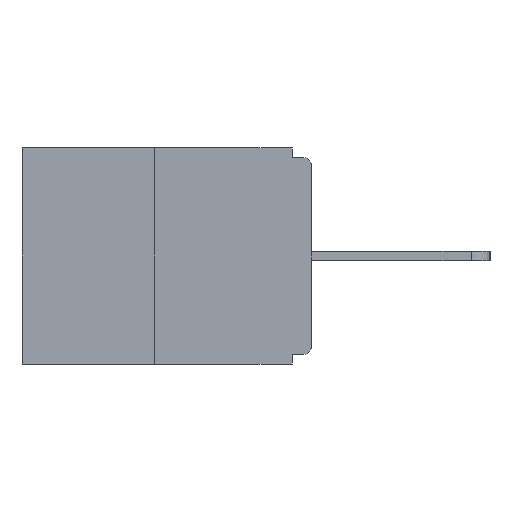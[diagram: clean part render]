
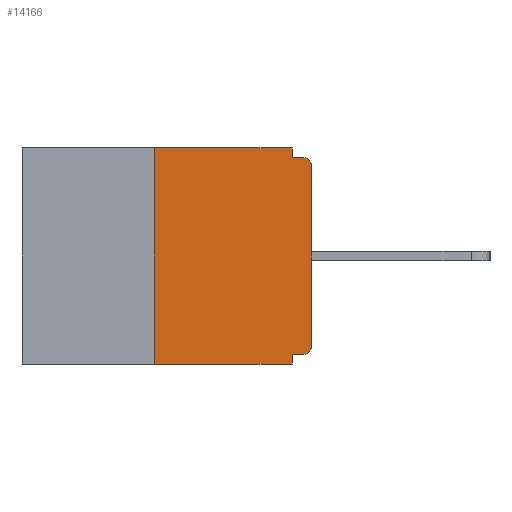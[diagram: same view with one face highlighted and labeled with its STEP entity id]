
A CAD part, left-side view. The second image highlights one B-rep face of the part: STEP entity #14166.
In plain terms, the highlighted planar face has unit normal (-1, 0, 0).
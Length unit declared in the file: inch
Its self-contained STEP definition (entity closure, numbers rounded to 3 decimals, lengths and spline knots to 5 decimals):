
#535 = CARTESIAN_POINT ( 'NONE',  ( 0., 0., 0. ) ) ;
#595 = AXIS2_PLACEMENT_3D ( 'NONE', #3139, #4774, #6117 ) ;
#619 = VERTEX_POINT ( 'NONE', #1560 ) ;
#704 = CARTESIAN_POINT ( 'NONE',  ( 0., 0.015, -0.328 ) ) ;
#728 = DIRECTION ( 'NONE',  ( -1., 0., 0. ) ) ;
#1107 = EDGE_CURVE ( 'NONE', #2534, #619, #13327, .T. ) ;
#1173 = DIRECTION ( 'NONE',  ( -1., 0., 0. ) ) ;
#1190 = ORIENTED_EDGE ( 'NONE', *, *, #6194, .F. ) ;
#1349 = EDGE_CURVE ( 'NONE', #9789, #619, #15164, .T. ) ;
#1560 = CARTESIAN_POINT ( 'NONE',  ( 0., 0.031, -0.343 ) ) ;
#1561 = EDGE_CURVE ( 'NONE', #7508, #14681, #6844, .T. ) ;
#1723 = DIRECTION ( 'NONE',  ( 0., 1., 0. ) ) ;
#1742 = CIRCLE ( 'NONE', #9476, 0.015 ) ;
#1920 = EDGE_CURVE ( 'NONE', #14076, #9789, #2983, .T. ) ;
#1926 = CARTESIAN_POINT ( 'NONE',  ( 0., 0.46, -0.343 ) ) ;
#2534 = VERTEX_POINT ( 'NONE', #5025 ) ;
#2983 = LINE ( 'NONE', #8063, #6265 ) ;
#3139 = CARTESIAN_POINT ( 'NONE',  ( 0., 0.46, 0. ) ) ;
#3207 = ORIENTED_EDGE ( 'NONE', *, *, #1561, .F. ) ;
#3322 = ORIENTED_EDGE ( 'NONE', *, *, #1107, .T. ) ;
#3447 = VECTOR ( 'NONE', #14392, 39.37008 ) ;
#4351 = VECTOR ( 'NONE', #5631, 39.37008 ) ;
#4774 = DIRECTION ( 'NONE',  ( 1., 0., 0. ) ) ;
#5005 = DIRECTION ( 'NONE',  ( 0., 0., -1. ) ) ;
#5025 = CARTESIAN_POINT ( 'NONE',  ( 0., 0.25, -0.343 ) ) ;
#5091 = CARTESIAN_POINT ( 'NONE',  ( 0., 0., -0.313 ) ) ;
#5329 = VECTOR ( 'NONE', #11363, 39.37008 ) ;
#5631 = DIRECTION ( 'NONE',  ( 0., 0., 1. ) ) ;
#5707 = ORIENTED_EDGE ( 'NONE', *, *, #15314, .T. ) ;
#5793 = CARTESIAN_POINT ( 'NONE',  ( 0., 0.25, 0. ) ) ;
#5821 = DIRECTION ( 'NONE',  ( 0., 0., -1. ) ) ;
#5864 = AXIS2_PLACEMENT_3D ( 'NONE', #10265, #1173, #5005 ) ;
#5916 = EDGE_LOOP ( 'NONE', ( #10541, #13088, #3322, #13416, #15775, #12745, #5707, #12383, #3207, #1190 ) ) ;
#5962 = VECTOR ( 'NONE', #10667, 39.37008 ) ;
#6117 = DIRECTION ( 'NONE',  ( 0., 0., -1. ) ) ;
#6194 = EDGE_CURVE ( 'NONE', #10847, #7508, #9401, .T. ) ;
#6265 = VECTOR ( 'NONE', #1723, 39.37008 ) ;
#6599 = VECTOR ( 'NONE', #6964, 39.37008 ) ;
#6844 = LINE ( 'NONE', #9334, #3447 ) ;
#6928 = CARTESIAN_POINT ( 'NONE',  ( 0., 0.031, -0.328 ) ) ;
#6964 = DIRECTION ( 'NONE',  ( 0., 0., 1. ) ) ;
#7444 = CARTESIAN_POINT ( 'NONE',  ( 0., 0.46, 0. ) ) ;
#7508 = VERTEX_POINT ( 'NONE', #15894 ) ;
#7604 = EDGE_CURVE ( 'NONE', #11170, #14681, #1742, .T. ) ;
#7662 = CARTESIAN_POINT ( 'NONE',  ( 0., 0.25, 0. ) ) ;
#8063 = CARTESIAN_POINT ( 'NONE',  ( 0., 0., -0.328 ) ) ;
#8158 = CARTESIAN_POINT ( 'NONE',  ( 0., 0.031, 0. ) ) ;
#8962 = EDGE_CURVE ( 'NONE', #2534, #9676, #13021, .T. ) ;
#9334 = CARTESIAN_POINT ( 'NONE',  ( 0., 0., -0.015 ) ) ;
#9401 = LINE ( 'NONE', #8158, #16071 ) ;
#9467 = FACE_OUTER_BOUND ( 'NONE', #5916, .T. ) ;
#9476 = AXIS2_PLACEMENT_3D ( 'NONE', #12057, #728, #5821 ) ;
#9590 = VECTOR ( 'NONE', #15416, 39.37008 ) ;
#9676 = VERTEX_POINT ( 'NONE', #7662 ) ;
#9789 = VERTEX_POINT ( 'NONE', #6928 ) ;
#10265 = CARTESIAN_POINT ( 'NONE',  ( 0., 0.015, -0.313 ) ) ;
#10541 = ORIENTED_EDGE ( 'NONE', *, *, #12144, .F. ) ;
#10667 = DIRECTION ( 'NONE',  ( 0., -1., 0. ) ) ;
#10847 = VERTEX_POINT ( 'NONE', #13826 ) ;
#10854 = VERTEX_POINT ( 'NONE', #5091 ) ;
#10956 = EDGE_CURVE ( 'NONE', #14076, #10854, #14902, .T. ) ;
#11170 = VERTEX_POINT ( 'NONE', #12154 ) ;
#11363 = DIRECTION ( 'NONE',  ( 0., -1., 0. ) ) ;
#12057 = CARTESIAN_POINT ( 'NONE',  ( 0., 0.015, -0.03 ) ) ;
#12144 = EDGE_CURVE ( 'NONE', #9676, #10847, #13770, .T. ) ;
#12154 = CARTESIAN_POINT ( 'NONE',  ( 0., 0., -0.03 ) ) ;
#12383 = ORIENTED_EDGE ( 'NONE', *, *, #7604, .T. ) ;
#12490 = CARTESIAN_POINT ( 'NONE',  ( 0., 0.031, -0.343 ) ) ;
#12745 = ORIENTED_EDGE ( 'NONE', *, *, #10956, .T. ) ;
#13021 = LINE ( 'NONE', #5793, #6599 ) ;
#13088 = ORIENTED_EDGE ( 'NONE', *, *, #8962, .F. ) ;
#13218 = DIRECTION ( 'NONE',  ( 0., 0., -1. ) ) ;
#13327 = LINE ( 'NONE', #1926, #5962 ) ;
#13416 = ORIENTED_EDGE ( 'NONE', *, *, #1349, .F. ) ;
#13529 = LINE ( 'NONE', #535, #4351 ) ;
#13770 = LINE ( 'NONE', #7444, #5329 ) ;
#13826 = CARTESIAN_POINT ( 'NONE',  ( 0., 0.031, 0. ) ) ;
#14076 = VERTEX_POINT ( 'NONE', #704 ) ;
#14166 = ADVANCED_FACE ( 'NONE', ( #9467 ), #14525, .F. ) ;
#14392 = DIRECTION ( 'NONE',  ( 0., -1., 0. ) ) ;
#14525 = PLANE ( 'NONE',  #595 ) ;
#14681 = VERTEX_POINT ( 'NONE', #16383 ) ;
#14902 = CIRCLE ( 'NONE', #5864, 0.015 ) ;
#15164 = LINE ( 'NONE', #12490, #9590 ) ;
#15314 = EDGE_CURVE ( 'NONE', #10854, #11170, #13529, .T. ) ;
#15416 = DIRECTION ( 'NONE',  ( 0., 0., -1. ) ) ;
#15775 = ORIENTED_EDGE ( 'NONE', *, *, #1920, .F. ) ;
#15894 = CARTESIAN_POINT ( 'NONE',  ( 0., 0.031, -0.015 ) ) ;
#16071 = VECTOR ( 'NONE', #13218, 39.37008 ) ;
#16383 = CARTESIAN_POINT ( 'NONE',  ( 0., 0.015, -0.015 ) ) ;
